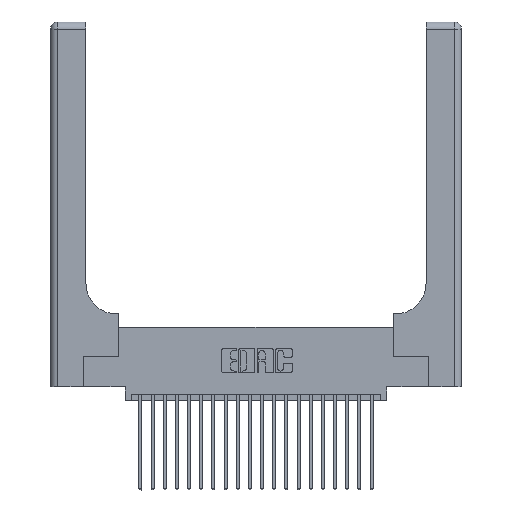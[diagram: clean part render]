
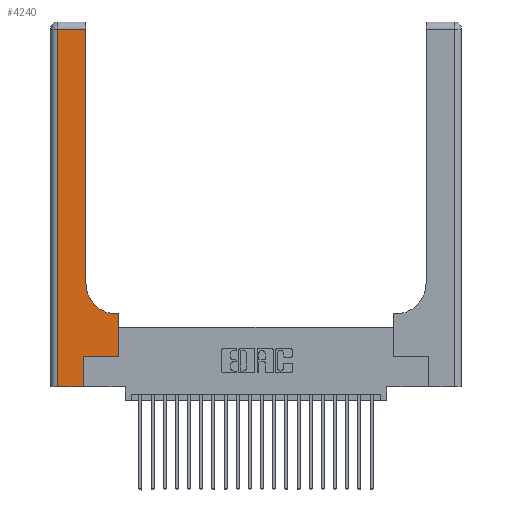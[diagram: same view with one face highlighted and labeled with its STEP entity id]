
A CAD part, top view. The second image highlights one B-rep face of the part: STEP entity #4240.
In plain terms, the highlighted planar face has unit normal (0, 0, 1).
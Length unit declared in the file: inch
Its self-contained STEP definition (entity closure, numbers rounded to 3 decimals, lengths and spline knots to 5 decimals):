
#86 = EDGE_CURVE ( 'NONE', #6946, #22968, #20159, .T. ) ;
#273 = LINE ( 'NONE', #13363, #19354 ) ;
#754 = LINE ( 'NONE', #6965, #9722 ) ;
#1048 = VECTOR ( 'NONE', #20451, 39.37008 ) ;
#1329 = DIRECTION ( 'NONE',  ( -1., 0., 0. ) ) ;
#1521 = CARTESIAN_POINT ( 'NONE',  ( 0.06, 3., 0.37 ) ) ;
#1647 = VERTEX_POINT ( 'NONE', #14109 ) ;
#2340 = CARTESIAN_POINT ( 'NONE',  ( 0.06, 2.94, 0.37 ) ) ;
#2500 = PLANE ( 'NONE',  #18927 ) ;
#2793 = VECTOR ( 'NONE', #5714, 39.37008 ) ;
#3223 = VERTEX_POINT ( 'NONE', #12683 ) ;
#3987 = EDGE_CURVE ( 'NONE', #1647, #3223, #17853, .T. ) ;
#4084 = AXIS2_PLACEMENT_3D ( 'NONE', #17148, #11914, #23053 ) ;
#4240 = ADVANCED_FACE ( 'NONE', ( #12905 ), #2500, .F. ) ;
#4287 = VECTOR ( 'NONE', #15369, 39.37008 ) ;
#4438 = VERTEX_POINT ( 'NONE', #2340 ) ;
#4552 = EDGE_CURVE ( 'NONE', #12829, #22676, #8591, .T. ) ;
#4908 = CARTESIAN_POINT ( 'NONE',  ( 0.2915, 2.94, 0.37 ) ) ;
#5550 = LINE ( 'NONE', #8700, #14759 ) ;
#5714 = DIRECTION ( 'NONE',  ( 1., 0., 0. ) ) ;
#5990 = LINE ( 'NONE', #22432, #1048 ) ;
#6946 = VERTEX_POINT ( 'NONE', #22024 ) ;
#6965 = CARTESIAN_POINT ( 'NONE',  ( 0.269, 0.25, 0.37 ) ) ;
#7005 = ORIENTED_EDGE ( 'NONE', *, *, #20491, .T. ) ;
#7109 = LINE ( 'NONE', #1521, #20662 ) ;
#7417 = CARTESIAN_POINT ( 'NONE',  ( 0.2915, 0.85, 0.37 ) ) ;
#8330 = ORIENTED_EDGE ( 'NONE', *, *, #18895, .T. ) ;
#8591 = CIRCLE ( 'NONE', #4084, 0.25 ) ;
#8640 = VECTOR ( 'NONE', #1329, 39.37008 ) ;
#8700 = CARTESIAN_POINT ( 'NONE',  ( 0.269, 0., 0.37 ) ) ;
#9035 = EDGE_CURVE ( 'NONE', #22968, #9734, #5550, .T. ) ;
#9197 = CARTESIAN_POINT ( 'NONE',  ( 0., 0., 0.37 ) ) ;
#9722 = VECTOR ( 'NONE', #19867, 39.37008 ) ;
#9734 = VERTEX_POINT ( 'NONE', #23750 ) ;
#9737 = CARTESIAN_POINT ( 'NONE',  ( 0.5585, 0.25, 0.37 ) ) ;
#11014 = EDGE_CURVE ( 'NONE', #22676, #15716, #273, .T. ) ;
#11824 = EDGE_CURVE ( 'NONE', #3223, #12829, #16446, .T. ) ;
#11914 = DIRECTION ( 'NONE',  ( 0., 0., -1. ) ) ;
#12119 = ORIENTED_EDGE ( 'NONE', *, *, #4552, .T. ) ;
#12150 = ORIENTED_EDGE ( 'NONE', *, *, #19474, .T. ) ;
#12259 = ORIENTED_EDGE ( 'NONE', *, *, #11824, .T. ) ;
#12683 = CARTESIAN_POINT ( 'NONE',  ( 0.5585, 0.6, 0.37 ) ) ;
#12829 = VERTEX_POINT ( 'NONE', #20933 ) ;
#12905 = FACE_OUTER_BOUND ( 'NONE', #18783, .T. ) ;
#13363 = CARTESIAN_POINT ( 'NONE',  ( 0.2915, 3., 0.37 ) ) ;
#13777 = DIRECTION ( 'NONE',  ( -1., 0., 0. ) ) ;
#14109 = CARTESIAN_POINT ( 'NONE',  ( 0.5585, 0.25, 0.37 ) ) ;
#14565 = ORIENTED_EDGE ( 'NONE', *, *, #86, .T. ) ;
#14759 = VECTOR ( 'NONE', #23619, 39.37008 ) ;
#15369 = DIRECTION ( 'NONE',  ( 0., 1., 0. ) ) ;
#15716 = VERTEX_POINT ( 'NONE', #4908 ) ;
#16446 = LINE ( 'NONE', #23520, #8640 ) ;
#16788 = ORIENTED_EDGE ( 'NONE', *, *, #3987, .T. ) ;
#17148 = CARTESIAN_POINT ( 'NONE',  ( 0.5415, 0.85, 0.37 ) ) ;
#17853 = LINE ( 'NONE', #9737, #4287 ) ;
#18041 = ORIENTED_EDGE ( 'NONE', *, *, #11014, .T. ) ;
#18783 = EDGE_LOOP ( 'NONE', ( #18041, #8330, #7005, #14565, #22166, #12150, #16788, #12259, #12119 ) ) ;
#18895 = EDGE_CURVE ( 'NONE', #15716, #4438, #5990, .T. ) ;
#18927 = AXIS2_PLACEMENT_3D ( 'NONE', #22911, #23231, #13777 ) ;
#19354 = VECTOR ( 'NONE', #20938, 39.37008 ) ;
#19474 = EDGE_CURVE ( 'NONE', #9734, #1647, #754, .T. ) ;
#19867 = DIRECTION ( 'NONE',  ( 1., 0., 0. ) ) ;
#20159 = LINE ( 'NONE', #9197, #2793 ) ;
#20181 = DIRECTION ( 'NONE',  ( 0., -1., 0. ) ) ;
#20451 = DIRECTION ( 'NONE',  ( -1., 0., 0. ) ) ;
#20491 = EDGE_CURVE ( 'NONE', #4438, #6946, #7109, .T. ) ;
#20662 = VECTOR ( 'NONE', #20181, 39.37008 ) ;
#20933 = CARTESIAN_POINT ( 'NONE',  ( 0.5415, 0.6, 0.37 ) ) ;
#20938 = DIRECTION ( 'NONE',  ( 0., 1., 0. ) ) ;
#21311 = CARTESIAN_POINT ( 'NONE',  ( 0.269, 0., 0.37 ) ) ;
#22024 = CARTESIAN_POINT ( 'NONE',  ( 0.06, 0., 0.37 ) ) ;
#22166 = ORIENTED_EDGE ( 'NONE', *, *, #9035, .T. ) ;
#22432 = CARTESIAN_POINT ( 'NONE',  ( 0., 2.94, 0.37 ) ) ;
#22676 = VERTEX_POINT ( 'NONE', #7417 ) ;
#22911 = CARTESIAN_POINT ( 'NONE',  ( 0., 3., 0.37 ) ) ;
#22968 = VERTEX_POINT ( 'NONE', #21311 ) ;
#23053 = DIRECTION ( 'NONE',  ( 1., 0., 0. ) ) ;
#23231 = DIRECTION ( 'NONE',  ( 0., 0., -1. ) ) ;
#23520 = CARTESIAN_POINT ( 'NONE',  ( 0.2915, 0.6, 0.37 ) ) ;
#23619 = DIRECTION ( 'NONE',  ( 0., 1., 0. ) ) ;
#23750 = CARTESIAN_POINT ( 'NONE',  ( 0.269, 0.25, 0.37 ) ) ;
